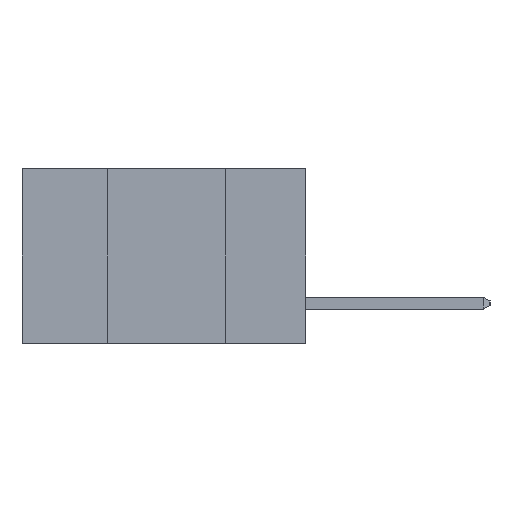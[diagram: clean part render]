
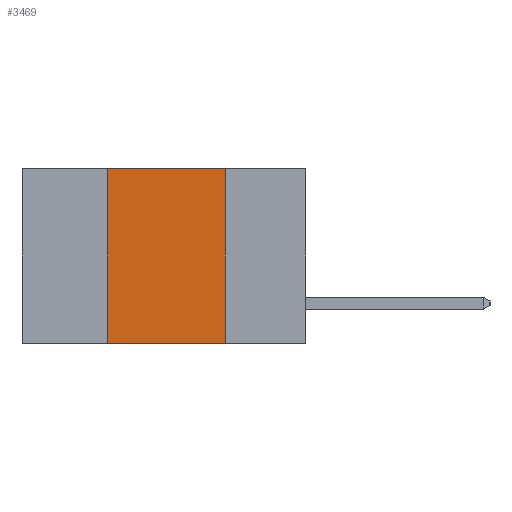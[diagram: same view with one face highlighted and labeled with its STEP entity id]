
A CAD part, left-side view. The second image highlights one B-rep face of the part: STEP entity #3469.
In plain terms, the highlighted planar face has unit normal (-1, 0, 0).
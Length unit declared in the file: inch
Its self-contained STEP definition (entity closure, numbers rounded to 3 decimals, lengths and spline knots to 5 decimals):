
#85 = CARTESIAN_POINT ( 'NONE',  ( 0., 0.42, 0. ) ) ;
#755 = ORIENTED_EDGE ( 'NONE', *, *, #11872, .F. ) ;
#769 = VERTEX_POINT ( 'NONE', #11047 ) ;
#1323 = ORIENTED_EDGE ( 'NONE', *, *, #2786, .F. ) ;
#2105 = ORIENTED_EDGE ( 'NONE', *, *, #4581, .T. ) ;
#2408 = DIRECTION ( 'NONE',  ( 0., 0., -1. ) ) ;
#2693 = DIRECTION ( 'NONE',  ( 0., 0., 1. ) ) ;
#2786 = EDGE_CURVE ( 'NONE', #11427, #769, #3592, .T. ) ;
#3197 = VECTOR ( 'NONE', #2408, 39.37008 ) ;
#3469 = ADVANCED_FACE ( 'NONE', ( #14091 ), #3566, .F. ) ;
#3566 = PLANE ( 'NONE',  #11198 ) ;
#3592 = LINE ( 'NONE', #3837, #3197 ) ;
#3618 = DIRECTION ( 'NONE',  ( 0., 0., -1. ) ) ;
#3632 = DIRECTION ( 'NONE',  ( 0., -1., 0. ) ) ;
#3664 = EDGE_CURVE ( 'NONE', #14719, #7039, #14623, .T. ) ;
#3675 = DIRECTION ( 'NONE',  ( 1., 0., 0. ) ) ;
#3837 = CARTESIAN_POINT ( 'NONE',  ( 0., 0.17, 0. ) ) ;
#4270 = LINE ( 'NONE', #13248, #13617 ) ;
#4412 = DIRECTION ( 'NONE',  ( 0., -1., 0. ) ) ;
#4581 = EDGE_CURVE ( 'NONE', #14719, #769, #4270, .T. ) ;
#5521 = EDGE_LOOP ( 'NONE', ( #1323, #755, #7171, #2105 ) ) ;
#6780 = VECTOR ( 'NONE', #4412, 39.37008 ) ;
#7039 = VERTEX_POINT ( 'NONE', #85 ) ;
#7171 = ORIENTED_EDGE ( 'NONE', *, *, #3664, .F. ) ;
#8302 = VECTOR ( 'NONE', #2693, 39.37008 ) ;
#9319 = CARTESIAN_POINT ( 'NONE',  ( 0., 0.6, 0. ) ) ;
#10978 = CARTESIAN_POINT ( 'NONE',  ( 0., 0.17, 0. ) ) ;
#11047 = CARTESIAN_POINT ( 'NONE',  ( 0., 0.17, -0.37 ) ) ;
#11198 = AXIS2_PLACEMENT_3D ( 'NONE', #14725, #3675, #3618 ) ;
#11427 = VERTEX_POINT ( 'NONE', #10978 ) ;
#11872 = EDGE_CURVE ( 'NONE', #7039, #11427, #13170, .T. ) ;
#13170 = LINE ( 'NONE', #9319, #6780 ) ;
#13248 = CARTESIAN_POINT ( 'NONE',  ( 0., 0.6, -0.37 ) ) ;
#13600 = CARTESIAN_POINT ( 'NONE',  ( 0., 0.42, 0. ) ) ;
#13617 = VECTOR ( 'NONE', #3632, 39.37008 ) ;
#14091 = FACE_OUTER_BOUND ( 'NONE', #5521, .T. ) ;
#14623 = LINE ( 'NONE', #13600, #8302 ) ;
#14719 = VERTEX_POINT ( 'NONE', #15496 ) ;
#14725 = CARTESIAN_POINT ( 'NONE',  ( 0., 0.6, 0. ) ) ;
#15496 = CARTESIAN_POINT ( 'NONE',  ( 0., 0.42, -0.37 ) ) ;
